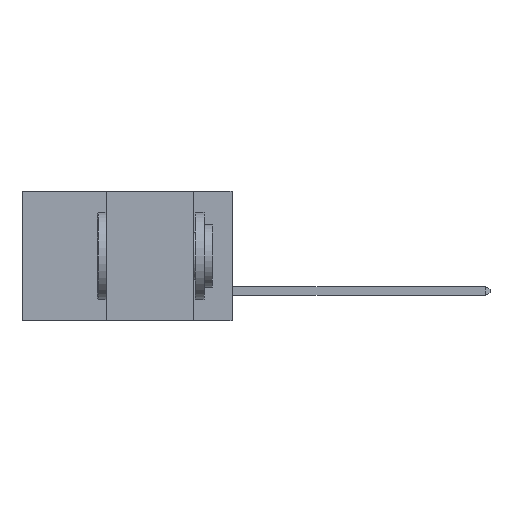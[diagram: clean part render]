
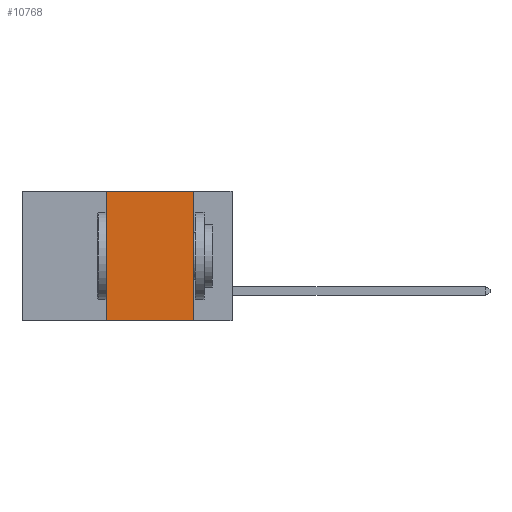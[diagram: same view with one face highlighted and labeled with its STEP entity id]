
A CAD part, left-side view. The second image highlights one B-rep face of the part: STEP entity #10768.
In plain terms, the highlighted planar face has unit normal (-1, 0, 0).
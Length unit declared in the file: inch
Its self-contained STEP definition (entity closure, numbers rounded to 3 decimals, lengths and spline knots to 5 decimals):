
#103 = EDGE_CURVE ( 'NONE', #13126, #3175, #1384, .T. ) ;
#1384 = LINE ( 'NONE', #22150, #17716 ) ;
#2024 = LINE ( 'NONE', #23691, #24650 ) ;
#2044 = CARTESIAN_POINT ( 'NONE',  ( 0., 0.6, 0. ) ) ;
#2065 = CARTESIAN_POINT ( 'NONE',  ( 0., 0.36, -0.37 ) ) ;
#2388 = ORIENTED_EDGE ( 'NONE', *, *, #103, .F. ) ;
#3175 = VERTEX_POINT ( 'NONE', #20594 ) ;
#3279 = LINE ( 'NONE', #21499, #8975 ) ;
#3392 = ORIENTED_EDGE ( 'NONE', *, *, #3430, .F. ) ;
#3430 = EDGE_CURVE ( 'NONE', #8593, #13126, #3279, .T. ) ;
#3803 = CARTESIAN_POINT ( 'NONE',  ( 0., 0.36, 0. ) ) ;
#3970 = VERTEX_POINT ( 'NONE', #14163 ) ;
#4199 = DIRECTION ( 'NONE',  ( 0., 0., -1. ) ) ;
#4680 = FACE_OUTER_BOUND ( 'NONE', #8381, .T. ) ;
#4774 = AXIS2_PLACEMENT_3D ( 'NONE', #2044, #16967, #4199 ) ;
#8175 = DIRECTION ( 'NONE',  ( 0., 0., 1. ) ) ;
#8381 = EDGE_LOOP ( 'NONE', ( #16113, #2388, #3392, #19757 ) ) ;
#8593 = VERTEX_POINT ( 'NONE', #2065 ) ;
#8975 = VECTOR ( 'NONE', #8175, 39.37008 ) ;
#9000 = LINE ( 'NONE', #16867, #25224 ) ;
#10768 = ADVANCED_FACE ( 'NONE', ( #4680 ), #27454, .F. ) ;
#11024 = DIRECTION ( 'NONE',  ( 0., -1., 0. ) ) ;
#13126 = VERTEX_POINT ( 'NONE', #3803 ) ;
#14163 = CARTESIAN_POINT ( 'NONE',  ( 0., 0.11, -0.37 ) ) ;
#16113 = ORIENTED_EDGE ( 'NONE', *, *, #22695, .F. ) ;
#16867 = CARTESIAN_POINT ( 'NONE',  ( 0., 0.11, 0. ) ) ;
#16967 = DIRECTION ( 'NONE',  ( 1., 0., 0. ) ) ;
#17716 = VECTOR ( 'NONE', #24254, 39.37008 ) ;
#18350 = EDGE_CURVE ( 'NONE', #8593, #3970, #2024, .T. ) ;
#19757 = ORIENTED_EDGE ( 'NONE', *, *, #18350, .T. ) ;
#20594 = CARTESIAN_POINT ( 'NONE',  ( 0., 0.11, 0. ) ) ;
#21499 = CARTESIAN_POINT ( 'NONE',  ( 0., 0.36, 0. ) ) ;
#22150 = CARTESIAN_POINT ( 'NONE',  ( 0., 0.6, 0. ) ) ;
#22695 = EDGE_CURVE ( 'NONE', #3175, #3970, #9000, .T. ) ;
#23691 = CARTESIAN_POINT ( 'NONE',  ( 0., 0.6, -0.37 ) ) ;
#24254 = DIRECTION ( 'NONE',  ( 0., -1., 0. ) ) ;
#24650 = VECTOR ( 'NONE', #11024, 39.37008 ) ;
#25224 = VECTOR ( 'NONE', #27358, 39.37008 ) ;
#27358 = DIRECTION ( 'NONE',  ( 0., 0., -1. ) ) ;
#27454 = PLANE ( 'NONE',  #4774 ) ;
